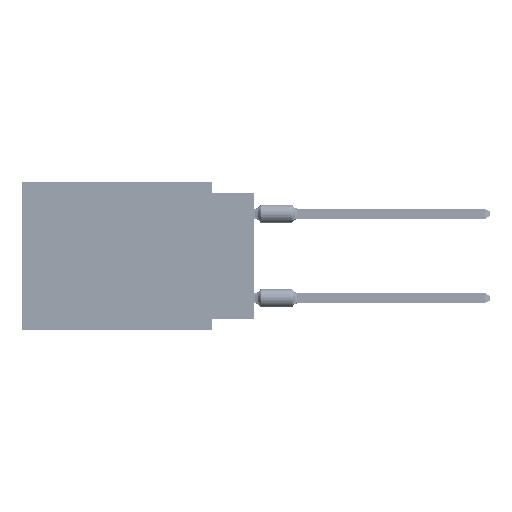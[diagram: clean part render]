
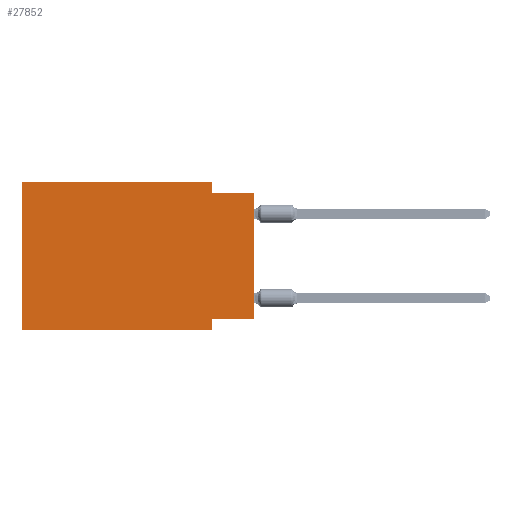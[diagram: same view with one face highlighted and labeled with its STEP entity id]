
A CAD part, left-side view. The second image highlights one B-rep face of the part: STEP entity #27852.
In plain terms, the highlighted planar face has unit normal (-1, 0, 0).
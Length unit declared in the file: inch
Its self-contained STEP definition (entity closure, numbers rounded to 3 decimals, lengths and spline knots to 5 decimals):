
#424 = LINE ( 'NONE', #42509, #63445 ) ;
#1658 = LINE ( 'NONE', #61470, #12518 ) ;
#2164 = AXIS2_PLACEMENT_3D ( 'NONE', #27253, #71202, #33572 ) ;
#2944 = VECTOR ( 'NONE', #79148, 39.37008 ) ;
#3298 = VERTEX_POINT ( 'NONE', #40122 ) ;
#4948 = CARTESIAN_POINT ( 'NONE',  ( 0., 0.55, -0.35 ) ) ;
#9606 = VECTOR ( 'NONE', #13388, 39.37008 ) ;
#10239 = VECTOR ( 'NONE', #73093, 39.37008 ) ;
#10565 = DIRECTION ( 'NONE',  ( 0., -1., 0. ) ) ;
#11185 = DIRECTION ( 'NONE',  ( 0., 0., -1. ) ) ;
#11476 = ORIENTED_EDGE ( 'NONE', *, *, #67900, .F. ) ;
#12271 = VECTOR ( 'NONE', #30294, 39.37008 ) ;
#12518 = VECTOR ( 'NONE', #11185, 39.37008 ) ;
#12790 = VERTEX_POINT ( 'NONE', #63314 ) ;
#13186 = ORIENTED_EDGE ( 'NONE', *, *, #41163, .F. ) ;
#13388 = DIRECTION ( 'NONE',  ( 0., 1., 0. ) ) ;
#16236 = CARTESIAN_POINT ( 'NONE',  ( 0., 0., 0. ) ) ;
#17083 = VECTOR ( 'NONE', #10565, 39.37008 ) ;
#17801 = LINE ( 'NONE', #73822, #49214 ) ;
#19861 = VERTEX_POINT ( 'NONE', #41873 ) ;
#20900 = PLANE ( 'NONE',  #2164 ) ;
#22932 = CARTESIAN_POINT ( 'NONE',  ( 0., 0., -0.025 ) ) ;
#23595 = EDGE_LOOP ( 'NONE', ( #44167, #11476, #81243, #35073, #50360, #49332, #36038, #13186 ) ) ;
#24888 = FACE_OUTER_BOUND ( 'NONE', #23595, .T. ) ;
#27253 = CARTESIAN_POINT ( 'NONE',  ( 0., 0.55, 0. ) ) ;
#27852 = ADVANCED_FACE ( 'NONE', ( #24888 ), #20900, .F. ) ;
#29172 = CARTESIAN_POINT ( 'NONE',  ( 0., 0.1, -0.35 ) ) ;
#30044 = VERTEX_POINT ( 'NONE', #43333 ) ;
#30294 = DIRECTION ( 'NONE',  ( 0., -1., 0. ) ) ;
#32971 = EDGE_CURVE ( 'NONE', #43621, #19861, #1658, .T. ) ;
#33572 = DIRECTION ( 'NONE',  ( 0., 0., -1. ) ) ;
#34439 = LINE ( 'NONE', #16236, #2944 ) ;
#35073 = ORIENTED_EDGE ( 'NONE', *, *, #53666, .F. ) ;
#36038 = ORIENTED_EDGE ( 'NONE', *, *, #70731, .F. ) ;
#36518 = CARTESIAN_POINT ( 'NONE',  ( 0., 0.55, -0.35 ) ) ;
#36977 = EDGE_CURVE ( 'NONE', #40310, #42220, #17801, .T. ) ;
#40122 = CARTESIAN_POINT ( 'NONE',  ( 0., 0., -0.025 ) ) ;
#40310 = VERTEX_POINT ( 'NONE', #36518 ) ;
#41163 = EDGE_CURVE ( 'NONE', #12790, #30044, #59769, .T. ) ;
#41873 = CARTESIAN_POINT ( 'NONE',  ( 0., 0.1, -0.025 ) ) ;
#42220 = VERTEX_POINT ( 'NONE', #70713 ) ;
#42434 = DIRECTION ( 'NONE',  ( 0., 0., 1. ) ) ;
#42509 = CARTESIAN_POINT ( 'NONE',  ( 0., 0.55, 0. ) ) ;
#43333 = CARTESIAN_POINT ( 'NONE',  ( 0., 0.1, -0.325 ) ) ;
#43621 = VERTEX_POINT ( 'NONE', #54812 ) ;
#44167 = ORIENTED_EDGE ( 'NONE', *, *, #46095, .T. ) ;
#46095 = EDGE_CURVE ( 'NONE', #12790, #3298, #34439, .T. ) ;
#49214 = VECTOR ( 'NONE', #42434, 39.37008 ) ;
#49332 = ORIENTED_EDGE ( 'NONE', *, *, #63320, .T. ) ;
#50360 = ORIENTED_EDGE ( 'NONE', *, *, #36977, .F. ) ;
#53666 = EDGE_CURVE ( 'NONE', #42220, #43621, #424, .T. ) ;
#54812 = CARTESIAN_POINT ( 'NONE',  ( 0., 0.1, 0. ) ) ;
#57344 = CARTESIAN_POINT ( 'NONE',  ( 0., 0., -0.325 ) ) ;
#58471 = LINE ( 'NONE', #4948, #12271 ) ;
#59769 = LINE ( 'NONE', #57344, #9606 ) ;
#61470 = CARTESIAN_POINT ( 'NONE',  ( 0., 0.1, 0. ) ) ;
#62149 = VERTEX_POINT ( 'NONE', #72400 ) ;
#63314 = CARTESIAN_POINT ( 'NONE',  ( 0., 0., -0.325 ) ) ;
#63320 = EDGE_CURVE ( 'NONE', #40310, #62149, #58471, .T. ) ;
#63445 = VECTOR ( 'NONE', #67616, 39.37008 ) ;
#67616 = DIRECTION ( 'NONE',  ( 0., -1., 0. ) ) ;
#67900 = EDGE_CURVE ( 'NONE', #19861, #3298, #69246, .T. ) ;
#69246 = LINE ( 'NONE', #22932, #17083 ) ;
#69251 = LINE ( 'NONE', #29172, #10239 ) ;
#70713 = CARTESIAN_POINT ( 'NONE',  ( 0., 0.55, 0. ) ) ;
#70731 = EDGE_CURVE ( 'NONE', #30044, #62149, #69251, .T. ) ;
#71202 = DIRECTION ( 'NONE',  ( 1., 0., 0. ) ) ;
#72400 = CARTESIAN_POINT ( 'NONE',  ( 0., 0.1, -0.35 ) ) ;
#73093 = DIRECTION ( 'NONE',  ( 0., 0., -1. ) ) ;
#73822 = CARTESIAN_POINT ( 'NONE',  ( 0., 0.55, 0. ) ) ;
#79148 = DIRECTION ( 'NONE',  ( 0., 0., 1. ) ) ;
#81243 = ORIENTED_EDGE ( 'NONE', *, *, #32971, .F. ) ;
